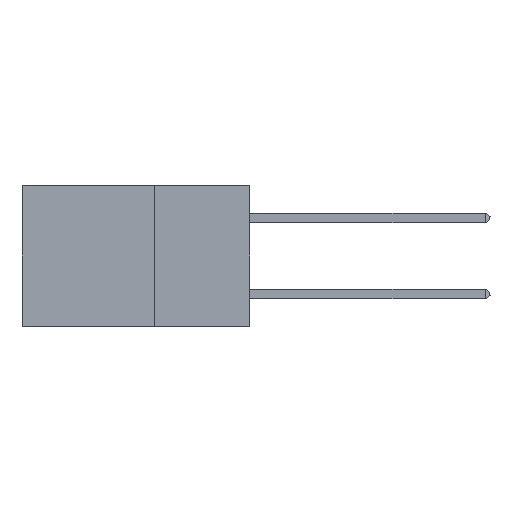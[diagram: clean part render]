
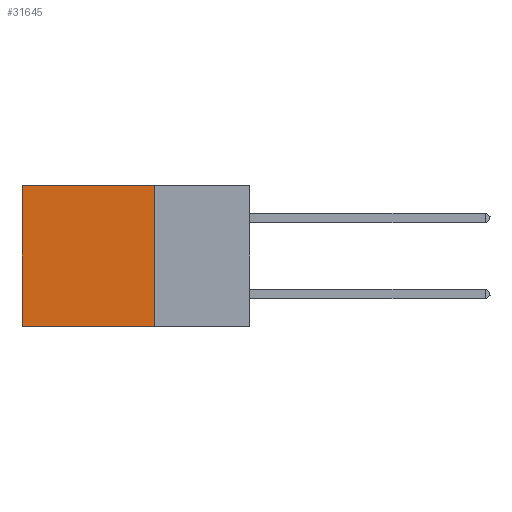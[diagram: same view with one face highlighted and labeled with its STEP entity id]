
A CAD part, left-side view. The second image highlights one B-rep face of the part: STEP entity #31645.
In plain terms, the highlighted planar face has unit normal (-1, 0, 0).
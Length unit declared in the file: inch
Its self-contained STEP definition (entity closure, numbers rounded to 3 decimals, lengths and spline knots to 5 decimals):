
#1317 = EDGE_LOOP ( 'NONE', ( #23309, #10953, #30921, #26335 ) ) ;
#2003 = CARTESIAN_POINT ( 'NONE',  ( 0.2875, 0.25, 0. ) ) ;
#2734 = VECTOR ( 'NONE', #16446, 39.37008 ) ;
#2793 = DIRECTION ( 'NONE',  ( 0., 1., 0. ) ) ;
#3122 = LINE ( 'NONE', #29961, #2734 ) ;
#4458 = DIRECTION ( 'NONE',  ( 0., 0., -1. ) ) ;
#4556 = CARTESIAN_POINT ( 'NONE',  ( 0.2875, 0.6, 0. ) ) ;
#5191 = VECTOR ( 'NONE', #2793, 39.37008 ) ;
#6673 = CARTESIAN_POINT ( 'NONE',  ( 0.2875, 0.25, 0. ) ) ;
#8731 = VERTEX_POINT ( 'NONE', #4556 ) ;
#9146 = EDGE_CURVE ( 'NONE', #15380, #28784, #29212, .T. ) ;
#10953 = ORIENTED_EDGE ( 'NONE', *, *, #22193, .F. ) ;
#11270 = LINE ( 'NONE', #24867, #32312 ) ;
#12290 = VECTOR ( 'NONE', #4458, 39.37008 ) ;
#12292 = EDGE_CURVE ( 'NONE', #8731, #30019, #11270, .T. ) ;
#12656 = DIRECTION ( 'NONE',  ( 1., 0., 0. ) ) ;
#14350 = PLANE ( 'NONE',  #21464 ) ;
#14801 = DIRECTION ( 'NONE',  ( 0., 0., -1. ) ) ;
#15380 = VERTEX_POINT ( 'NONE', #6673 ) ;
#16446 = DIRECTION ( 'NONE',  ( 0., 1., 0. ) ) ;
#21464 = AXIS2_PLACEMENT_3D ( 'NONE', #2003, #12656, #32784 ) ;
#21619 = EDGE_CURVE ( 'NONE', #15380, #8731, #3122, .T. ) ;
#22193 = EDGE_CURVE ( 'NONE', #28784, #30019, #33257, .T. ) ;
#23112 = CARTESIAN_POINT ( 'NONE',  ( 0.2875, 0.25, -0.37 ) ) ;
#23254 = CARTESIAN_POINT ( 'NONE',  ( 0.2875, 0.25, 0. ) ) ;
#23309 = ORIENTED_EDGE ( 'NONE', *, *, #12292, .T. ) ;
#24867 = CARTESIAN_POINT ( 'NONE',  ( 0.2875, 0.6, 0. ) ) ;
#25422 = CARTESIAN_POINT ( 'NONE',  ( 0.2875, 0.6, -0.37 ) ) ;
#26335 = ORIENTED_EDGE ( 'NONE', *, *, #21619, .T. ) ;
#26703 = CARTESIAN_POINT ( 'NONE',  ( 0.2875, 0.25, -0.37 ) ) ;
#28784 = VERTEX_POINT ( 'NONE', #23112 ) ;
#29212 = LINE ( 'NONE', #23254, #12290 ) ;
#29961 = CARTESIAN_POINT ( 'NONE',  ( 0.2875, 0.25, 0. ) ) ;
#30019 = VERTEX_POINT ( 'NONE', #25422 ) ;
#30921 = ORIENTED_EDGE ( 'NONE', *, *, #9146, .F. ) ;
#31645 = ADVANCED_FACE ( 'NONE', ( #32734 ), #14350, .F. ) ;
#32312 = VECTOR ( 'NONE', #14801, 39.37008 ) ;
#32734 = FACE_OUTER_BOUND ( 'NONE', #1317, .T. ) ;
#32784 = DIRECTION ( 'NONE',  ( 0., 0., -1. ) ) ;
#33257 = LINE ( 'NONE', #26703, #5191 ) ;
